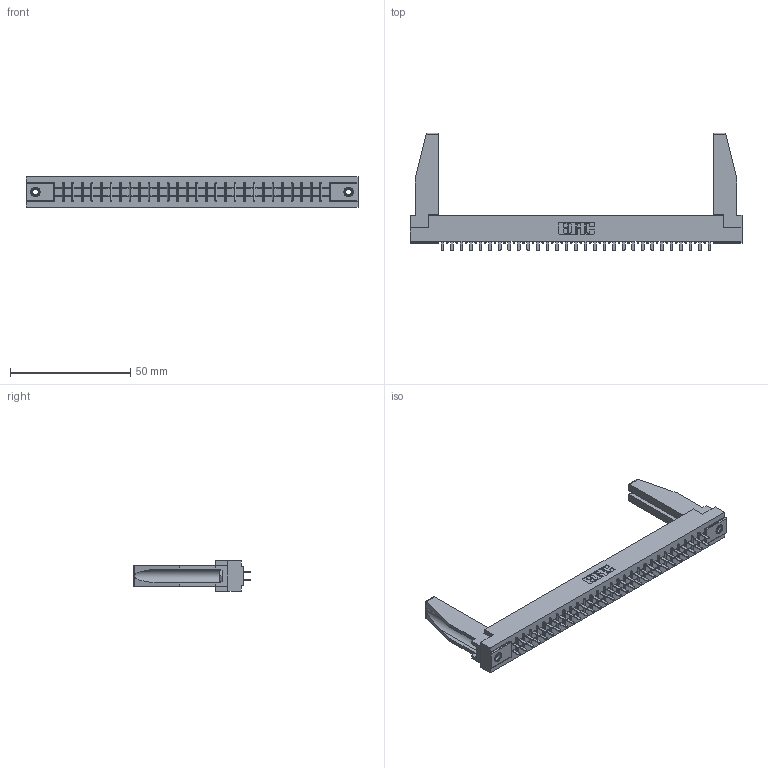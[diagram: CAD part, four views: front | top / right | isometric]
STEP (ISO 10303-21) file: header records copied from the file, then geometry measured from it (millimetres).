
FILE_DESCRIPTION (( 'STEP AP203' ), '1' );
FILE_NAME ('315-058-521-278.STEP', '2019-09-10T19:44:57', ( '' ), ( '' ), 'SwSTEP 2.0', 'SolidWorks 2016', '' );
FILE_SCHEMA (( 'CONFIG_CONTROL_DESIGN' ));
Length unit declared in the file: inch
Products named in the file (5): 315-058-521-278; 305-290-001_521; 307-220-078; 305 Part_.156 Dia; 345-250-001_345-250-001-102
Assembly tree (63 placements, depth 2):
  315-058-521-278
    305 Part_.156 Dia
    305-290-001_521  x58
    345-250-001_345-250-001-102  x2
    307-220-078  x2
Bounding box: 137.92 x 48.9 x 12.7 mm (x, y, z)
Volume: 18254 mm3; surface area: 21386.7 mm2
Topology: 63 solids, 63 shells, 2914 faces, 8273 edges, 5350 vertices
Faces by surface type: plane 1718, cylinder 1064, sphere 116, cone 12, torus 4
Entity records: 35301 total; most frequent: CARTESIAN_POINT 5847, ORIENTED_EDGE 5760, DIRECTION 5624, EDGE_CURVE 2880, VECTOR 2314, LINE 2314, VERTEX_POINT 1836, AXIS2_PLACEMENT_3D 1655
